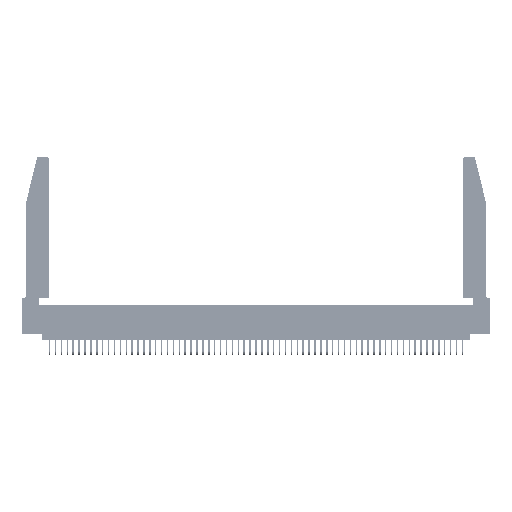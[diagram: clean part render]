
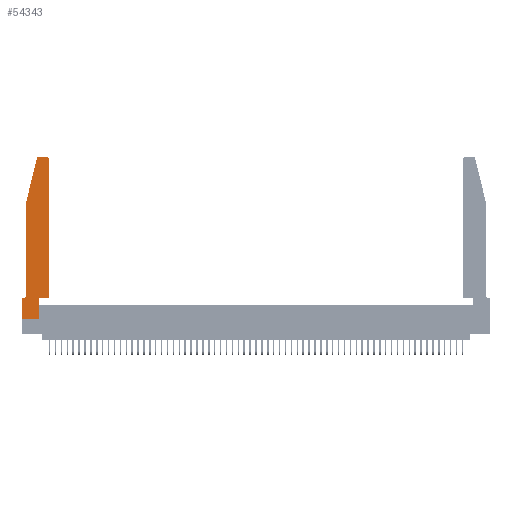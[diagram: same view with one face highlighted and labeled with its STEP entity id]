
A CAD part, top view. The second image highlights one B-rep face of the part: STEP entity #54343.
In plain terms, the highlighted planar face has unit normal (0, 0, 1).
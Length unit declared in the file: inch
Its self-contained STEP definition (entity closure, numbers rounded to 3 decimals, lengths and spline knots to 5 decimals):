
#194 = DIRECTION ( 'NONE',  ( 0., 0., 1. ) ) ;
#514 = VERTEX_POINT ( 'NONE', #33001 ) ;
#2373 = VERTEX_POINT ( 'NONE', #37568 ) ;
#2486 = LINE ( 'NONE', #47532, #25153 ) ;
#3290 = DIRECTION ( 'NONE',  ( 1., 0., 0. ) ) ;
#3412 = CIRCLE ( 'NONE', #26102, 0.03 ) ;
#3442 = VECTOR ( 'NONE', #20528, 39.37008 ) ;
#3572 = DIRECTION ( 'NONE',  ( 0., 0., -1. ) ) ;
#5776 = LINE ( 'NONE', #30261, #52247 ) ;
#6053 = DIRECTION ( 'NONE',  ( -1., 0., 0. ) ) ;
#6140 = VERTEX_POINT ( 'NONE', #33853 ) ;
#6298 = ORIENTED_EDGE ( 'NONE', *, *, #23984, .T. ) ;
#6725 = CARTESIAN_POINT ( 'NONE',  ( 0.25487, 2.72718, 0.37 ) ) ;
#8533 = EDGE_CURVE ( 'NONE', #47097, #514, #42603, .T. ) ;
#10513 = VECTOR ( 'NONE', #35438, 39.37008 ) ;
#10855 = EDGE_CURVE ( 'NONE', #16053, #47097, #27498, .T. ) ;
#10954 = VECTOR ( 'NONE', #12182, 39.37008 ) ;
#12182 = DIRECTION ( 'NONE',  ( 0., 1., 0. ) ) ;
#14158 = VECTOR ( 'NONE', #6053, 39.37008 ) ;
#15421 = EDGE_CURVE ( 'NONE', #38092, #38511, #31613, .T. ) ;
#15554 = DIRECTION ( 'NONE',  ( -0.239, -0.971, 0. ) ) ;
#16053 = VERTEX_POINT ( 'NONE', #30228 ) ;
#16939 = CARTESIAN_POINT ( 'NONE',  ( 0., 0., 0.37 ) ) ;
#16980 = ORIENTED_EDGE ( 'NONE', *, *, #49734, .T. ) ;
#17260 = CARTESIAN_POINT ( 'NONE',  ( 0.2605, 2.75, 0.37 ) ) ;
#17574 = CIRCLE ( 'NONE', #24781, 0.03 ) ;
#18085 = FACE_OUTER_BOUND ( 'NONE', #56502, .T. ) ;
#19227 = CARTESIAN_POINT ( 'NONE',  ( 0., 0.35, 0.37 ) ) ;
#20528 = DIRECTION ( 'NONE',  ( 0., -1., 0. ) ) ;
#21315 = ORIENTED_EDGE ( 'NONE', *, *, #27382, .T. ) ;
#21799 = CARTESIAN_POINT ( 'NONE',  ( 0.0755, 2., 0.37 ) ) ;
#22307 = CARTESIAN_POINT ( 'NONE',  ( 0.0755, 0.42, 0.37 ) ) ;
#22671 = ORIENTED_EDGE ( 'NONE', *, *, #30788, .T. ) ;
#23739 = DIRECTION ( 'NONE',  ( 0., 0., 1. ) ) ;
#23984 = EDGE_CURVE ( 'NONE', #51803, #38092, #5776, .T. ) ;
#24781 = AXIS2_PLACEMENT_3D ( 'NONE', #57229, #30401, #3290 ) ;
#25153 = VECTOR ( 'NONE', #52008, 39.37008 ) ;
#25586 = EDGE_CURVE ( 'NONE', #53192, #44318, #3412, .T. ) ;
#26102 = AXIS2_PLACEMENT_3D ( 'NONE', #27343, #194, #31909 ) ;
#26162 = LINE ( 'NONE', #41951, #14158 ) ;
#27343 = CARTESIAN_POINT ( 'NONE',  ( 0.284, 2.72, 0.37 ) ) ;
#27382 = EDGE_CURVE ( 'NONE', #6140, #56676, #41462, .T. ) ;
#27498 = LINE ( 'NONE', #33943, #3442 ) ;
#28167 = EDGE_CURVE ( 'NONE', #38511, #16053, #26162, .T. ) ;
#28244 = ORIENTED_EDGE ( 'NONE', *, *, #8533, .T. ) ;
#28572 = CARTESIAN_POINT ( 'NONE',  ( 0.2865, 0.35, 0.37 ) ) ;
#30228 = CARTESIAN_POINT ( 'NONE',  ( 0., 0.35, 0.37 ) ) ;
#30261 = CARTESIAN_POINT ( 'NONE',  ( 0.0755, 2., 0.37 ) ) ;
#30350 = LINE ( 'NONE', #38050, #52786 ) ;
#30401 = DIRECTION ( 'NONE',  ( 0., 0., 1. ) ) ;
#30644 = VECTOR ( 'NONE', #50135, 39.37008 ) ;
#30683 = CARTESIAN_POINT ( 'NONE',  ( 0.0055, 0.42, 0.37 ) ) ;
#30788 = EDGE_CURVE ( 'NONE', #42983, #6140, #2486, .T. ) ;
#31613 = CIRCLE ( 'NONE', #32605, 0.07 ) ;
#31909 = DIRECTION ( 'NONE',  ( 1., 0., 0. ) ) ;
#32605 = AXIS2_PLACEMENT_3D ( 'NONE', #30683, #3572, #35266 ) ;
#33001 = CARTESIAN_POINT ( 'NONE',  ( 0.2865, 0., 0.37 ) ) ;
#33853 = CARTESIAN_POINT ( 'NONE',  ( 0.4505, 0.35, 0.37 ) ) ;
#33943 = CARTESIAN_POINT ( 'NONE',  ( 0., 0., 0.37 ) ) ;
#35266 = DIRECTION ( 'NONE',  ( -1., 0., 0. ) ) ;
#35438 = DIRECTION ( 'NONE',  ( -1., 0., 0. ) ) ;
#36181 = CARTESIAN_POINT ( 'NONE',  ( 0.4505, 2.72, 0.37 ) ) ;
#36443 = LINE ( 'NONE', #48205, #10954 ) ;
#37568 = CARTESIAN_POINT ( 'NONE',  ( 0.4205, 2.75, 0.37 ) ) ;
#38050 = CARTESIAN_POINT ( 'NONE',  ( 0.0755, 2., 0.37 ) ) ;
#38082 = ORIENTED_EDGE ( 'NONE', *, *, #47784, .T. ) ;
#38092 = VERTEX_POINT ( 'NONE', #22307 ) ;
#38511 = VERTEX_POINT ( 'NONE', #47420 ) ;
#41462 = LINE ( 'NONE', #55084, #51931 ) ;
#41650 = ORIENTED_EDGE ( 'NONE', *, *, #28167, .T. ) ;
#41859 = EDGE_CURVE ( 'NONE', #44318, #51803, #30350, .T. ) ;
#41951 = CARTESIAN_POINT ( 'NONE',  ( 0.0755, 0.35, 0.37 ) ) ;
#42579 = EDGE_CURVE ( 'NONE', #56676, #2373, #17574, .T. ) ;
#42603 = LINE ( 'NONE', #53913, #30644 ) ;
#42983 = VERTEX_POINT ( 'NONE', #28572 ) ;
#44318 = VERTEX_POINT ( 'NONE', #6725 ) ;
#44717 = ORIENTED_EDGE ( 'NONE', *, *, #42579, .T. ) ;
#44875 = CARTESIAN_POINT ( 'NONE',  ( 0.284, 2.75, 0.37 ) ) ;
#46132 = DIRECTION ( 'NONE',  ( 0., 1., 0. ) ) ;
#46908 = ORIENTED_EDGE ( 'NONE', *, *, #25586, .T. ) ;
#47030 = AXIS2_PLACEMENT_3D ( 'NONE', #19227, #23739, #55119 ) ;
#47097 = VERTEX_POINT ( 'NONE', #16939 ) ;
#47420 = CARTESIAN_POINT ( 'NONE',  ( 0.0055, 0.35, 0.37 ) ) ;
#47532 = CARTESIAN_POINT ( 'NONE',  ( 0.4505, 0.35, 0.37 ) ) ;
#47784 = EDGE_CURVE ( 'NONE', #2373, #53192, #58326, .T. ) ;
#48205 = CARTESIAN_POINT ( 'NONE',  ( 0.2865, 0.35, 0.37 ) ) ;
#48300 = DIRECTION ( 'NONE',  ( 0., -1., 0. ) ) ;
#49734 = EDGE_CURVE ( 'NONE', #514, #42983, #36443, .T. ) ;
#50135 = DIRECTION ( 'NONE',  ( 1., 0., 0. ) ) ;
#50661 = PLANE ( 'NONE',  #47030 ) ;
#50853 = ORIENTED_EDGE ( 'NONE', *, *, #15421, .T. ) ;
#51803 = VERTEX_POINT ( 'NONE', #21799 ) ;
#51931 = VECTOR ( 'NONE', #46132, 39.37008 ) ;
#52008 = DIRECTION ( 'NONE',  ( 1., 0., 0. ) ) ;
#52247 = VECTOR ( 'NONE', #48300, 39.37008 ) ;
#52786 = VECTOR ( 'NONE', #15554, 39.37008 ) ;
#53192 = VERTEX_POINT ( 'NONE', #44875 ) ;
#53913 = CARTESIAN_POINT ( 'NONE',  ( 0., 0., 0.37 ) ) ;
#54343 = ADVANCED_FACE ( 'NONE', ( #18085 ), #50661, .T. ) ;
#54492 = ORIENTED_EDGE ( 'NONE', *, *, #41859, .T. ) ;
#55084 = CARTESIAN_POINT ( 'NONE',  ( 0.4505, 0.35, 0.37 ) ) ;
#55119 = DIRECTION ( 'NONE',  ( 1., 0., 0. ) ) ;
#56502 = EDGE_LOOP ( 'NONE', ( #38082, #46908, #54492, #6298, #50853, #41650, #56573, #28244, #16980, #22671, #21315, #44717 ) ) ;
#56573 = ORIENTED_EDGE ( 'NONE', *, *, #10855, .T. ) ;
#56676 = VERTEX_POINT ( 'NONE', #36181 ) ;
#57229 = CARTESIAN_POINT ( 'NONE',  ( 0.4205, 2.72, 0.37 ) ) ;
#58326 = LINE ( 'NONE', #17260, #10513 ) ;
